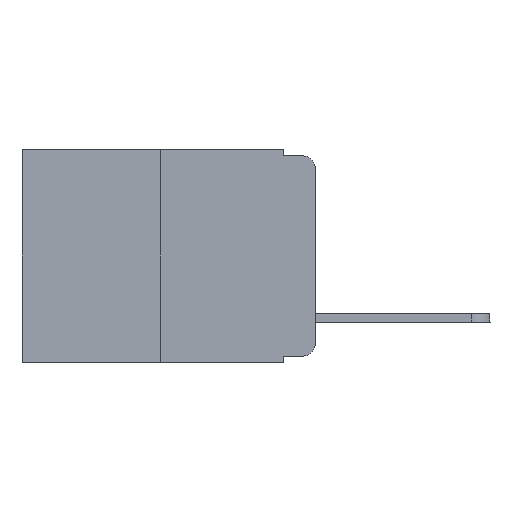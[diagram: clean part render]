
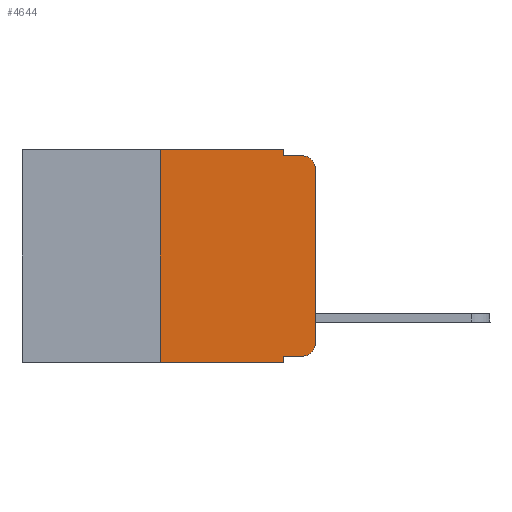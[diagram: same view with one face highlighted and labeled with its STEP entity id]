
A CAD part, left-side view. The second image highlights one B-rep face of the part: STEP entity #4644.
In plain terms, the highlighted planar face has unit normal (-1, 0, 0).
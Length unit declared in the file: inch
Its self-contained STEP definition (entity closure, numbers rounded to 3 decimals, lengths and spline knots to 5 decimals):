
#230 = ORIENTED_EDGE ( 'NONE', *, *, #2855, .F. ) ;
#628 = LINE ( 'NONE', #13297, #12138 ) ;
#1037 = CARTESIAN_POINT ( 'NONE',  ( 0., 0., 0. ) ) ;
#1470 = EDGE_CURVE ( 'NONE', #7648, #4808, #628, .T. ) ;
#1541 = VECTOR ( 'NONE', #7971, 39.37008 ) ;
#1719 = CARTESIAN_POINT ( 'NONE',  ( 0., 0.02, -0.313 ) ) ;
#1740 = FACE_OUTER_BOUND ( 'NONE', #11098, .T. ) ;
#1743 = VERTEX_POINT ( 'NONE', #2864 ) ;
#1758 = EDGE_CURVE ( 'NONE', #7082, #9023, #11948, .T. ) ;
#1864 = CARTESIAN_POINT ( 'NONE',  ( 0., 0.25, -0.343 ) ) ;
#2152 = CARTESIAN_POINT ( 'NONE',  ( 0., 0.25, 0. ) ) ;
#2168 = VERTEX_POINT ( 'NONE', #13033 ) ;
#2247 = DIRECTION ( 'NONE',  ( 0., 0., -1. ) ) ;
#2459 = CARTESIAN_POINT ( 'NONE',  ( 0., 0.051, -0.01 ) ) ;
#2471 = LINE ( 'NONE', #8230, #14544 ) ;
#2528 = VERTEX_POINT ( 'NONE', #3538 ) ;
#2557 = CARTESIAN_POINT ( 'NONE',  ( 0., 0.02, -0.03 ) ) ;
#2578 = ORIENTED_EDGE ( 'NONE', *, *, #13778, .T. ) ;
#2655 = DIRECTION ( 'NONE',  ( 0., -1., 0. ) ) ;
#2704 = AXIS2_PLACEMENT_3D ( 'NONE', #6870, #14013, #2247 ) ;
#2760 = PLANE ( 'NONE',  #2704 ) ;
#2834 = ORIENTED_EDGE ( 'NONE', *, *, #10612, .F. ) ;
#2855 = EDGE_CURVE ( 'NONE', #2168, #9819, #4165, .T. ) ;
#2864 = CARTESIAN_POINT ( 'NONE',  ( 0., 0., -0.03 ) ) ;
#3196 = CARTESIAN_POINT ( 'NONE',  ( 0., 0.051, 0. ) ) ;
#3538 = CARTESIAN_POINT ( 'NONE',  ( 0., 0.02, -0.01 ) ) ;
#3578 = DIRECTION ( 'NONE',  ( -1., 0., 0. ) ) ;
#3653 = EDGE_CURVE ( 'NONE', #4808, #7593, #6129, .T. ) ;
#4165 = LINE ( 'NONE', #3196, #13512 ) ;
#4294 = LINE ( 'NONE', #1037, #1541 ) ;
#4379 = CARTESIAN_POINT ( 'NONE',  ( 0., 0.051, -0.343 ) ) ;
#4644 = ADVANCED_FACE ( 'NONE', ( #1740 ), #2760, .F. ) ;
#4702 = DIRECTION ( 'NONE',  ( 0., 0., 1. ) ) ;
#4808 = VERTEX_POINT ( 'NONE', #6691 ) ;
#5148 = EDGE_CURVE ( 'NONE', #9819, #2528, #12341, .T. ) ;
#5242 = DIRECTION ( 'NONE',  ( -1., 0., 0. ) ) ;
#5435 = CIRCLE ( 'NONE', #11471, 0.02 ) ;
#5799 = CARTESIAN_POINT ( 'NONE',  ( 0., 0.473, 0. ) ) ;
#6061 = VECTOR ( 'NONE', #12876, 39.37008 ) ;
#6129 = CIRCLE ( 'NONE', #9835, 0.02 ) ;
#6658 = ORIENTED_EDGE ( 'NONE', *, *, #1758, .T. ) ;
#6691 = CARTESIAN_POINT ( 'NONE',  ( 0., 0.02, -0.333 ) ) ;
#6817 = VECTOR ( 'NONE', #4702, 39.37008 ) ;
#6870 = CARTESIAN_POINT ( 'NONE',  ( 0., 0.473, 0. ) ) ;
#6923 = DIRECTION ( 'NONE',  ( 0., -1., 0. ) ) ;
#6989 = LINE ( 'NONE', #11686, #6817 ) ;
#7046 = ORIENTED_EDGE ( 'NONE', *, *, #3653, .T. ) ;
#7082 = VERTEX_POINT ( 'NONE', #1864 ) ;
#7095 = DIRECTION ( 'NONE',  ( 0., 0., -1. ) ) ;
#7521 = VECTOR ( 'NONE', #13234, 39.37008 ) ;
#7593 = VERTEX_POINT ( 'NONE', #13263 ) ;
#7648 = VERTEX_POINT ( 'NONE', #12252 ) ;
#7971 = DIRECTION ( 'NONE',  ( 0., 0., 1. ) ) ;
#7977 = EDGE_CURVE ( 'NONE', #1743, #2528, #5435, .T. ) ;
#8230 = CARTESIAN_POINT ( 'NONE',  ( 0., 0.051, 0. ) ) ;
#8359 = CARTESIAN_POINT ( 'NONE',  ( 0., 0.051, -0.01 ) ) ;
#8454 = CARTESIAN_POINT ( 'NONE',  ( 0., 0.473, -0.343 ) ) ;
#8838 = VECTOR ( 'NONE', #6923, 39.37008 ) ;
#9023 = VERTEX_POINT ( 'NONE', #4379 ) ;
#9177 = ORIENTED_EDGE ( 'NONE', *, *, #1470, .T. ) ;
#9819 = VERTEX_POINT ( 'NONE', #2459 ) ;
#9835 = AXIS2_PLACEMENT_3D ( 'NONE', #1719, #5242, #14453 ) ;
#10129 = ORIENTED_EDGE ( 'NONE', *, *, #13871, .F. ) ;
#10612 = EDGE_CURVE ( 'NONE', #7648, #9023, #2471, .T. ) ;
#10963 = ORIENTED_EDGE ( 'NONE', *, *, #7977, .T. ) ;
#11098 = EDGE_LOOP ( 'NONE', ( #2578, #10963, #14624, #230, #12784, #10129, #6658, #2834, #9177, #7046 ) ) ;
#11184 = EDGE_CURVE ( 'NONE', #11795, #2168, #11971, .T. ) ;
#11471 = AXIS2_PLACEMENT_3D ( 'NONE', #2557, #3578, #11728 ) ;
#11686 = CARTESIAN_POINT ( 'NONE',  ( 0., 0.25, 0. ) ) ;
#11728 = DIRECTION ( 'NONE',  ( 0., 0., -1. ) ) ;
#11795 = VERTEX_POINT ( 'NONE', #2152 ) ;
#11948 = LINE ( 'NONE', #8454, #7521 ) ;
#11971 = LINE ( 'NONE', #5799, #8838 ) ;
#12138 = VECTOR ( 'NONE', #2655, 39.37008 ) ;
#12252 = CARTESIAN_POINT ( 'NONE',  ( 0., 0.051, -0.333 ) ) ;
#12341 = LINE ( 'NONE', #8359, #6061 ) ;
#12784 = ORIENTED_EDGE ( 'NONE', *, *, #11184, .F. ) ;
#12876 = DIRECTION ( 'NONE',  ( 0., -1., 0. ) ) ;
#13033 = CARTESIAN_POINT ( 'NONE',  ( 0., 0.051, 0. ) ) ;
#13234 = DIRECTION ( 'NONE',  ( 0., -1., 0. ) ) ;
#13263 = CARTESIAN_POINT ( 'NONE',  ( 0., 0., -0.313 ) ) ;
#13297 = CARTESIAN_POINT ( 'NONE',  ( 0., 0.051, -0.333 ) ) ;
#13512 = VECTOR ( 'NONE', #14636, 39.37008 ) ;
#13778 = EDGE_CURVE ( 'NONE', #7593, #1743, #4294, .T. ) ;
#13871 = EDGE_CURVE ( 'NONE', #7082, #11795, #6989, .T. ) ;
#14013 = DIRECTION ( 'NONE',  ( 1., 0., 0. ) ) ;
#14453 = DIRECTION ( 'NONE',  ( 0., 0., -1. ) ) ;
#14544 = VECTOR ( 'NONE', #7095, 39.37008 ) ;
#14624 = ORIENTED_EDGE ( 'NONE', *, *, #5148, .F. ) ;
#14636 = DIRECTION ( 'NONE',  ( 0., 0., -1. ) ) ;
